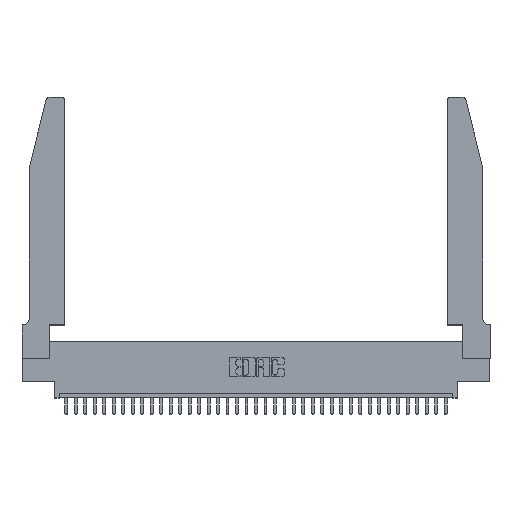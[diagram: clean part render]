
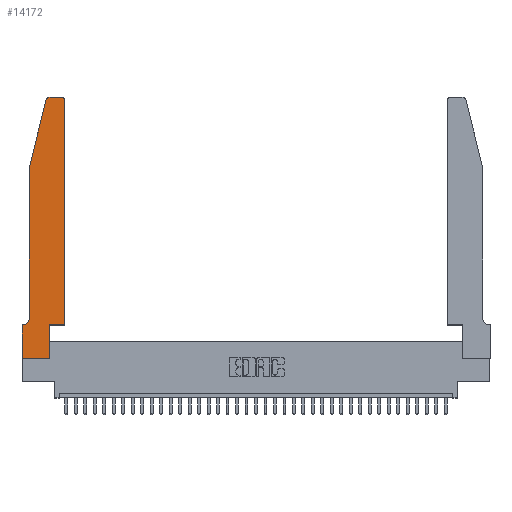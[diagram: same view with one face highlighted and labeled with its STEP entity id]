
A CAD part, top view. The second image highlights one B-rep face of the part: STEP entity #14172.
In plain terms, the highlighted planar face has unit normal (0, 0, 1).
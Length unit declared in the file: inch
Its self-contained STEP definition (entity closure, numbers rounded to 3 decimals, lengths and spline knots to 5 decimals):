
#125 = VERTEX_POINT ( 'NONE', #3069 ) ;
#654 = FACE_OUTER_BOUND ( 'NONE', #25822, .T. ) ;
#789 = CARTESIAN_POINT ( 'NONE',  ( 0.2605, 2.75, 0.37 ) ) ;
#860 = EDGE_CURVE ( 'NONE', #35672, #4390, #13745, .T. ) ;
#1846 = LINE ( 'NONE', #2471, #22301 ) ;
#2471 = CARTESIAN_POINT ( 'NONE',  ( 0., 0., 0.37 ) ) ;
#2515 = DIRECTION ( 'NONE',  ( -1., 0., 0. ) ) ;
#3069 = CARTESIAN_POINT ( 'NONE',  ( 0.4505, 0.35, 0.37 ) ) ;
#3557 = ORIENTED_EDGE ( 'NONE', *, *, #19922, .T. ) ;
#3704 = EDGE_CURVE ( 'NONE', #14316, #7351, #1846, .T. ) ;
#3790 = DIRECTION ( 'NONE',  ( 0., 1., 0. ) ) ;
#3856 = CARTESIAN_POINT ( 'NONE',  ( 0., 0.35, 0.37 ) ) ;
#4077 = DIRECTION ( 'NONE',  ( 0., 0., 1. ) ) ;
#4181 = ORIENTED_EDGE ( 'NONE', *, *, #12066, .T. ) ;
#4390 = VERTEX_POINT ( 'NONE', #9081 ) ;
#4433 = ORIENTED_EDGE ( 'NONE', *, *, #860, .T. ) ;
#4698 = LINE ( 'NONE', #30007, #14197 ) ;
#5853 = CARTESIAN_POINT ( 'NONE',  ( 0.0755, 2., 0.37 ) ) ;
#6736 = ORIENTED_EDGE ( 'NONE', *, *, #10131, .T. ) ;
#6981 = DIRECTION ( 'NONE',  ( 0., -1., 0. ) ) ;
#7125 = CIRCLE ( 'NONE', #17129, 0.07 ) ;
#7351 = VERTEX_POINT ( 'NONE', #24852 ) ;
#7737 = DIRECTION ( 'NONE',  ( 0., 0., -1. ) ) ;
#7924 = DIRECTION ( 'NONE',  ( 1., 0., 0. ) ) ;
#8093 = CARTESIAN_POINT ( 'NONE',  ( 0.0055, 0.42, 0.37 ) ) ;
#8778 = CARTESIAN_POINT ( 'NONE',  ( 0.2865, 0., 0.37 ) ) ;
#8942 = EDGE_CURVE ( 'NONE', #34423, #14316, #4698, .T. ) ;
#9081 = CARTESIAN_POINT ( 'NONE',  ( 0.4205, 2.75, 0.37 ) ) ;
#9298 = DIRECTION ( 'NONE',  ( 0., 1., 0. ) ) ;
#9611 = CARTESIAN_POINT ( 'NONE',  ( 0.4505, 2.72, 0.37 ) ) ;
#9662 = VECTOR ( 'NONE', #25193, 39.37008 ) ;
#9978 = VERTEX_POINT ( 'NONE', #8778 ) ;
#10131 = EDGE_CURVE ( 'NONE', #30942, #14782, #34564, .T. ) ;
#10868 = VECTOR ( 'NONE', #31111, 39.37008 ) ;
#10991 = ORIENTED_EDGE ( 'NONE', *, *, #13885, .T. ) ;
#11265 = AXIS2_PLACEMENT_3D ( 'NONE', #25423, #4077, #17048 ) ;
#11379 = LINE ( 'NONE', #5853, #9662 ) ;
#11854 = CARTESIAN_POINT ( 'NONE',  ( 0.4505, 0.35, 0.37 ) ) ;
#11968 = CARTESIAN_POINT ( 'NONE',  ( 0.2865, 0.35, 0.37 ) ) ;
#12066 = EDGE_CURVE ( 'NONE', #14782, #34423, #7125, .T. ) ;
#12324 = LINE ( 'NONE', #789, #16197 ) ;
#12410 = LINE ( 'NONE', #11854, #31929 ) ;
#12491 = VERTEX_POINT ( 'NONE', #16264 ) ;
#12956 = LINE ( 'NONE', #11968, #18137 ) ;
#13745 = CIRCLE ( 'NONE', #20172, 0.03 ) ;
#13872 = ORIENTED_EDGE ( 'NONE', *, *, #19429, .T. ) ;
#13885 = EDGE_CURVE ( 'NONE', #12491, #125, #32034, .T. ) ;
#14172 = ADVANCED_FACE ( 'NONE', ( #654 ), #25231, .T. ) ;
#14197 = VECTOR ( 'NONE', #2515, 39.37008 ) ;
#14316 = VERTEX_POINT ( 'NONE', #3856 ) ;
#14782 = VERTEX_POINT ( 'NONE', #29103 ) ;
#14825 = DIRECTION ( 'NONE',  ( -1., 0., 0. ) ) ;
#15151 = EDGE_CURVE ( 'NONE', #125, #35672, #12410, .T. ) ;
#15660 = DIRECTION ( 'NONE',  ( 0., 0., 1. ) ) ;
#16197 = VECTOR ( 'NONE', #14825, 39.37008 ) ;
#16264 = CARTESIAN_POINT ( 'NONE',  ( 0.2865, 0.35, 0.37 ) ) ;
#17048 = DIRECTION ( 'NONE',  ( 1., 0., 0. ) ) ;
#17129 = AXIS2_PLACEMENT_3D ( 'NONE', #8093, #7737, #24520 ) ;
#17153 = CARTESIAN_POINT ( 'NONE',  ( 0., 0., 0.37 ) ) ;
#17519 = ORIENTED_EDGE ( 'NONE', *, *, #31085, .T. ) ;
#18137 = VECTOR ( 'NONE', #9298, 39.37008 ) ;
#18438 = EDGE_CURVE ( 'NONE', #7351, #9978, #23878, .T. ) ;
#18705 = ORIENTED_EDGE ( 'NONE', *, *, #8942, .T. ) ;
#19235 = VERTEX_POINT ( 'NONE', #21150 ) ;
#19269 = AXIS2_PLACEMENT_3D ( 'NONE', #22153, #15660, #26107 ) ;
#19429 = EDGE_CURVE ( 'NONE', #9978, #12491, #12956, .T. ) ;
#19922 = EDGE_CURVE ( 'NONE', #4390, #24552, #12324, .T. ) ;
#20172 = AXIS2_PLACEMENT_3D ( 'NONE', #32686, #24578, #7924 ) ;
#21150 = CARTESIAN_POINT ( 'NONE',  ( 0.25487, 2.72718, 0.37 ) ) ;
#21889 = DIRECTION ( 'NONE',  ( 1., 0., 0. ) ) ;
#22153 = CARTESIAN_POINT ( 'NONE',  ( 0., 0.35, 0.37 ) ) ;
#22301 = VECTOR ( 'NONE', #27512, 39.37008 ) ;
#22799 = CARTESIAN_POINT ( 'NONE',  ( 0.4505, 0.35, 0.37 ) ) ;
#22890 = ORIENTED_EDGE ( 'NONE', *, *, #3704, .T. ) ;
#22918 = CIRCLE ( 'NONE', #11265, 0.03 ) ;
#23878 = LINE ( 'NONE', #17153, #10868 ) ;
#24520 = DIRECTION ( 'NONE',  ( -1., 0., 0. ) ) ;
#24552 = VERTEX_POINT ( 'NONE', #30673 ) ;
#24578 = DIRECTION ( 'NONE',  ( 0., 0., 1. ) ) ;
#24852 = CARTESIAN_POINT ( 'NONE',  ( 0., 0., 0.37 ) ) ;
#25193 = DIRECTION ( 'NONE',  ( -0.239, -0.971, 0. ) ) ;
#25231 = PLANE ( 'NONE',  #19269 ) ;
#25423 = CARTESIAN_POINT ( 'NONE',  ( 0.284, 2.72, 0.37 ) ) ;
#25558 = ORIENTED_EDGE ( 'NONE', *, *, #15151, .T. ) ;
#25822 = EDGE_LOOP ( 'NONE', ( #3557, #17519, #35301, #6736, #4181, #18705, #22890, #30856, #13872, #10991, #25558, #4433 ) ) ;
#26107 = DIRECTION ( 'NONE',  ( 1., 0., 0. ) ) ;
#27512 = DIRECTION ( 'NONE',  ( 0., -1., 0. ) ) ;
#27515 = CARTESIAN_POINT ( 'NONE',  ( 0.0755, 2., 0.37 ) ) ;
#28005 = VECTOR ( 'NONE', #6981, 39.37008 ) ;
#28371 = EDGE_CURVE ( 'NONE', #19235, #30942, #11379, .T. ) ;
#29103 = CARTESIAN_POINT ( 'NONE',  ( 0.0755, 0.42, 0.37 ) ) ;
#30007 = CARTESIAN_POINT ( 'NONE',  ( 0.0755, 0.35, 0.37 ) ) ;
#30673 = CARTESIAN_POINT ( 'NONE',  ( 0.284, 2.75, 0.37 ) ) ;
#30856 = ORIENTED_EDGE ( 'NONE', *, *, #18438, .T. ) ;
#30942 = VERTEX_POINT ( 'NONE', #27515 ) ;
#31085 = EDGE_CURVE ( 'NONE', #24552, #19235, #22918, .T. ) ;
#31111 = DIRECTION ( 'NONE',  ( 1., 0., 0. ) ) ;
#31929 = VECTOR ( 'NONE', #3790, 39.37008 ) ;
#32034 = LINE ( 'NONE', #22799, #32482 ) ;
#32115 = CARTESIAN_POINT ( 'NONE',  ( 0.0055, 0.35, 0.37 ) ) ;
#32482 = VECTOR ( 'NONE', #21889, 39.37008 ) ;
#32686 = CARTESIAN_POINT ( 'NONE',  ( 0.4205, 2.72, 0.37 ) ) ;
#34423 = VERTEX_POINT ( 'NONE', #32115 ) ;
#34564 = LINE ( 'NONE', #34658, #28005 ) ;
#34658 = CARTESIAN_POINT ( 'NONE',  ( 0.0755, 2., 0.37 ) ) ;
#35301 = ORIENTED_EDGE ( 'NONE', *, *, #28371, .T. ) ;
#35672 = VERTEX_POINT ( 'NONE', #9611 ) ;
